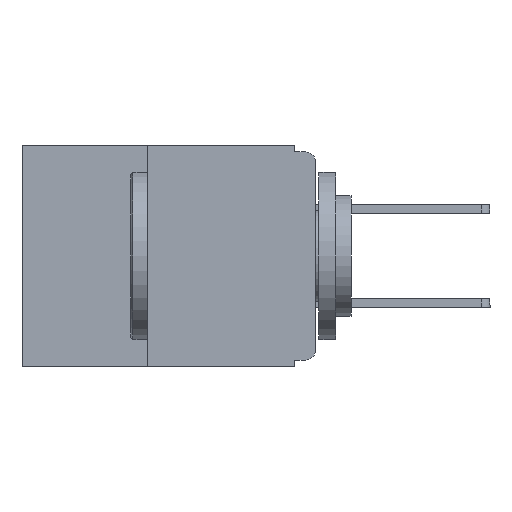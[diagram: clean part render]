
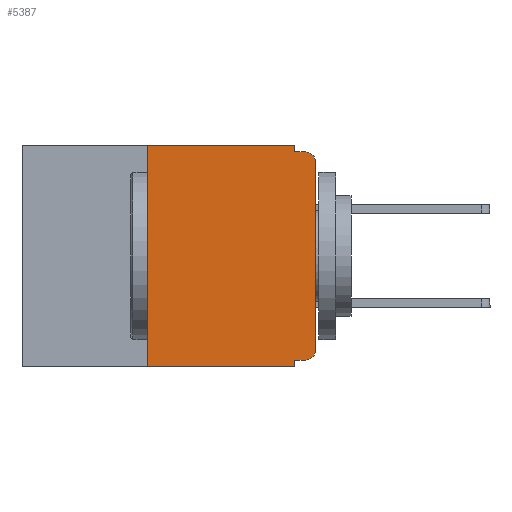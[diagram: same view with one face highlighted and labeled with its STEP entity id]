
A CAD part, left-side view. The second image highlights one B-rep face of the part: STEP entity #5387.
In plain terms, the highlighted planar face has unit normal (-1, 0, 0).
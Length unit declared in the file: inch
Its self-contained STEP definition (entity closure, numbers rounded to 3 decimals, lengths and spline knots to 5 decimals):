
#81 = ORIENTED_EDGE ( 'NONE', *, *, #3796, .T. ) ;
#101 = VERTEX_POINT ( 'NONE', #12151 ) ;
#143 = EDGE_CURVE ( 'NONE', #101, #3013, #11389, .T. ) ;
#520 = DIRECTION ( 'NONE',  ( 0., 0., 1. ) ) ;
#745 = VECTOR ( 'NONE', #13741, 39.37008 ) ;
#1279 = EDGE_CURVE ( 'NONE', #9571, #3043, #8392, .T. ) ;
#1328 = ORIENTED_EDGE ( 'NONE', *, *, #9820, .F. ) ;
#1627 = CARTESIAN_POINT ( 'NONE',  ( 0., 0.031, -0.32 ) ) ;
#2290 = CARTESIAN_POINT ( 'NONE',  ( 0., 0.015, -0.01 ) ) ;
#3013 = VERTEX_POINT ( 'NONE', #2290 ) ;
#3043 = VERTEX_POINT ( 'NONE', #7533 ) ;
#3123 = ORIENTED_EDGE ( 'NONE', *, *, #10642, .T. ) ;
#3796 = EDGE_CURVE ( 'NONE', #23147, #11884, #3865, .T. ) ;
#3861 = CARTESIAN_POINT ( 'NONE',  ( 0., 0., 0. ) ) ;
#3865 = CIRCLE ( 'NONE', #9009, 0.015 ) ;
#3958 = VECTOR ( 'NONE', #4576, 39.37008 ) ;
#4079 = CARTESIAN_POINT ( 'NONE',  ( 0., 0., -0.305 ) ) ;
#4576 = DIRECTION ( 'NONE',  ( 0., -1., 0. ) ) ;
#4621 = VERTEX_POINT ( 'NONE', #22062 ) ;
#4714 = LINE ( 'NONE', #19530, #22528 ) ;
#5159 = CIRCLE ( 'NONE', #9457, 0.015 ) ;
#5387 = ADVANCED_FACE ( 'NONE', ( #7196 ), #20436, .F. ) ;
#5475 = VECTOR ( 'NONE', #5738, 39.37008 ) ;
#5738 = DIRECTION ( 'NONE',  ( 0., 0., 1. ) ) ;
#6290 = VECTOR ( 'NONE', #17651, 39.37008 ) ;
#7161 = CARTESIAN_POINT ( 'NONE',  ( 0., 0.25, -0.33 ) ) ;
#7196 = FACE_OUTER_BOUND ( 'NONE', #7732, .T. ) ;
#7533 = CARTESIAN_POINT ( 'NONE',  ( 0., 0.031, 0. ) ) ;
#7732 = EDGE_LOOP ( 'NONE', ( #18998, #3123, #14790, #23779, #11137, #22101, #12796, #12638, #1328, #81 ) ) ;
#8185 = DIRECTION ( 'NONE',  ( 0., 0., -1. ) ) ;
#8190 = DIRECTION ( 'NONE',  ( -1., 0., 0. ) ) ;
#8392 = LINE ( 'NONE', #16141, #3958 ) ;
#8527 = CARTESIAN_POINT ( 'NONE',  ( 0., 0.015, -0.32 ) ) ;
#8779 = CARTESIAN_POINT ( 'NONE',  ( 0., 0.25, 0. ) ) ;
#9009 = AXIS2_PLACEMENT_3D ( 'NONE', #19657, #8190, #8185 ) ;
#9457 = AXIS2_PLACEMENT_3D ( 'NONE', #9757, #22436, #11644 ) ;
#9571 = VERTEX_POINT ( 'NONE', #8779 ) ;
#9757 = CARTESIAN_POINT ( 'NONE',  ( 0., 0.015, -0.025 ) ) ;
#9820 = EDGE_CURVE ( 'NONE', #23147, #12985, #21344, .T. ) ;
#9891 = VECTOR ( 'NONE', #520, 39.37008 ) ;
#10441 = VERTEX_POINT ( 'NONE', #7161 ) ;
#10642 = EDGE_CURVE ( 'NONE', #4621, #3013, #5159, .T. ) ;
#11137 = ORIENTED_EDGE ( 'NONE', *, *, #1279, .F. ) ;
#11279 = EDGE_CURVE ( 'NONE', #10441, #9571, #20124, .T. ) ;
#11334 = LINE ( 'NONE', #21184, #6290 ) ;
#11389 = LINE ( 'NONE', #16296, #745 ) ;
#11644 = DIRECTION ( 'NONE',  ( 0., 0., -1. ) ) ;
#11732 = VECTOR ( 'NONE', #18429, 39.37008 ) ;
#11884 = VERTEX_POINT ( 'NONE', #4079 ) ;
#12151 = CARTESIAN_POINT ( 'NONE',  ( 0., 0.031, -0.01 ) ) ;
#12638 = ORIENTED_EDGE ( 'NONE', *, *, #22551, .F. ) ;
#12738 = EDGE_CURVE ( 'NONE', #3043, #101, #11334, .T. ) ;
#12796 = ORIENTED_EDGE ( 'NONE', *, *, #23377, .T. ) ;
#12985 = VERTEX_POINT ( 'NONE', #1627 ) ;
#13551 = VECTOR ( 'NONE', #14875, 39.37008 ) ;
#13741 = DIRECTION ( 'NONE',  ( 0., -1., 0. ) ) ;
#14790 = ORIENTED_EDGE ( 'NONE', *, *, #143, .F. ) ;
#14875 = DIRECTION ( 'NONE',  ( 0., -1., 0. ) ) ;
#15779 = VERTEX_POINT ( 'NONE', #22273 ) ;
#16141 = CARTESIAN_POINT ( 'NONE',  ( 0., 0.437, 0. ) ) ;
#16296 = CARTESIAN_POINT ( 'NONE',  ( 0., 0., -0.01 ) ) ;
#16599 = CARTESIAN_POINT ( 'NONE',  ( 0., 0., -0.32 ) ) ;
#17651 = DIRECTION ( 'NONE',  ( 0., 0., -1. ) ) ;
#17806 = AXIS2_PLACEMENT_3D ( 'NONE', #20755, #20342, #20313 ) ;
#18316 = LINE ( 'NONE', #21992, #13551 ) ;
#18429 = DIRECTION ( 'NONE',  ( 0., 1., 0. ) ) ;
#18447 = EDGE_CURVE ( 'NONE', #11884, #4621, #20178, .T. ) ;
#18998 = ORIENTED_EDGE ( 'NONE', *, *, #18447, .T. ) ;
#19530 = CARTESIAN_POINT ( 'NONE',  ( 0., 0.031, -0.33 ) ) ;
#19657 = CARTESIAN_POINT ( 'NONE',  ( 0., 0.015, -0.305 ) ) ;
#20124 = LINE ( 'NONE', #22639, #9891 ) ;
#20178 = LINE ( 'NONE', #3861, #5475 ) ;
#20313 = DIRECTION ( 'NONE',  ( 0., 0., -1. ) ) ;
#20342 = DIRECTION ( 'NONE',  ( 1., 0., 0. ) ) ;
#20436 = PLANE ( 'NONE',  #17806 ) ;
#20755 = CARTESIAN_POINT ( 'NONE',  ( 0., 0.437, 0. ) ) ;
#21184 = CARTESIAN_POINT ( 'NONE',  ( 0., 0.031, 0. ) ) ;
#21330 = DIRECTION ( 'NONE',  ( 0., 0., -1. ) ) ;
#21344 = LINE ( 'NONE', #16599, #11732 ) ;
#21992 = CARTESIAN_POINT ( 'NONE',  ( 0., 0.437, -0.33 ) ) ;
#22062 = CARTESIAN_POINT ( 'NONE',  ( 0., 0., -0.025 ) ) ;
#22101 = ORIENTED_EDGE ( 'NONE', *, *, #11279, .F. ) ;
#22273 = CARTESIAN_POINT ( 'NONE',  ( 0., 0.031, -0.33 ) ) ;
#22436 = DIRECTION ( 'NONE',  ( -1., 0., 0. ) ) ;
#22528 = VECTOR ( 'NONE', #21330, 39.37008 ) ;
#22551 = EDGE_CURVE ( 'NONE', #12985, #15779, #4714, .T. ) ;
#22639 = CARTESIAN_POINT ( 'NONE',  ( 0., 0.25, -0.33 ) ) ;
#23147 = VERTEX_POINT ( 'NONE', #8527 ) ;
#23377 = EDGE_CURVE ( 'NONE', #10441, #15779, #18316, .T. ) ;
#23779 = ORIENTED_EDGE ( 'NONE', *, *, #12738, .F. ) ;
